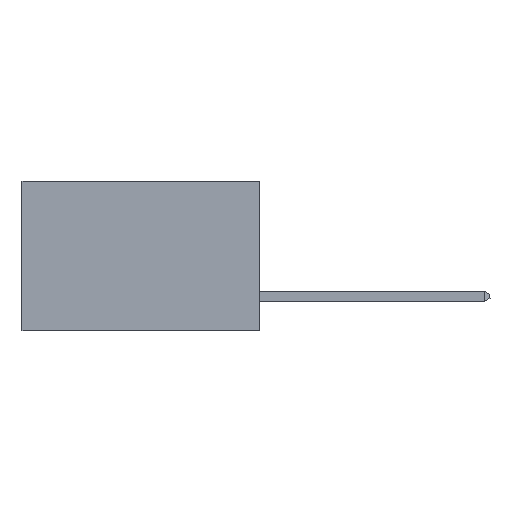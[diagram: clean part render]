
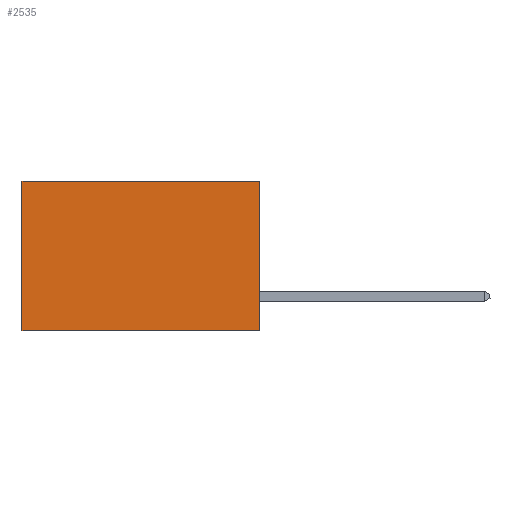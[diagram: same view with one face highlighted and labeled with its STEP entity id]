
A CAD part, left-side view. The second image highlights one B-rep face of the part: STEP entity #2535.
In plain terms, the highlighted planar face has unit normal (-1, 0, 0).
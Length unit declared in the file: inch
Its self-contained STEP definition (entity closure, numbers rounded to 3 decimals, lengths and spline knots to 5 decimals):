
#740 = VECTOR ( 'NONE', #2702, 39.37008 ) ;
#1398 = AXIS2_PLACEMENT_3D ( 'NONE', #10653, #1428, #5856 ) ;
#1407 = ORIENTED_EDGE ( 'NONE', *, *, #13389, .T. ) ;
#1428 = DIRECTION ( 'NONE',  ( 1., 0., 0. ) ) ;
#1784 = DIRECTION ( 'NONE',  ( 0., 1., 0. ) ) ;
#2108 = EDGE_CURVE ( 'NONE', #3399, #7770, #3367, .T. ) ;
#2535 = ADVANCED_FACE ( 'NONE', ( #5545 ), #6294, .F. ) ;
#2702 = DIRECTION ( 'NONE',  ( 0., 0., -1. ) ) ;
#2729 = VECTOR ( 'NONE', #1784, 39.37008 ) ;
#3332 = CARTESIAN_POINT ( 'NONE',  ( 0.277, 0.59, -0.37 ) ) ;
#3367 = LINE ( 'NONE', #5558, #4013 ) ;
#3399 = VERTEX_POINT ( 'NONE', #13139 ) ;
#3533 = DIRECTION ( 'NONE',  ( 0., 1., 0. ) ) ;
#3624 = LINE ( 'NONE', #6316, #740 ) ;
#4013 = VECTOR ( 'NONE', #3533, 39.37008 ) ;
#4144 = EDGE_CURVE ( 'NONE', #13652, #3399, #3624, .T. ) ;
#5545 = FACE_OUTER_BOUND ( 'NONE', #10223, .T. ) ;
#5558 = CARTESIAN_POINT ( 'NONE',  ( 0.277, 0., -0.37 ) ) ;
#5582 = LINE ( 'NONE', #12353, #2729 ) ;
#5856 = DIRECTION ( 'NONE',  ( 0., 0., -1. ) ) ;
#6294 = PLANE ( 'NONE',  #1398 ) ;
#6316 = CARTESIAN_POINT ( 'NONE',  ( 0.277, 0., -0.37 ) ) ;
#7189 = LINE ( 'NONE', #3332, #10255 ) ;
#7770 = VERTEX_POINT ( 'NONE', #10559 ) ;
#8631 = DIRECTION ( 'NONE',  ( 0., 0., -1. ) ) ;
#8984 = CARTESIAN_POINT ( 'NONE',  ( 0.277, 0., 0. ) ) ;
#10072 = CARTESIAN_POINT ( 'NONE',  ( 0.277, 0.59, 0. ) ) ;
#10223 = EDGE_LOOP ( 'NONE', ( #1407, #11291, #11586, #13709 ) ) ;
#10255 = VECTOR ( 'NONE', #8631, 39.37008 ) ;
#10559 = CARTESIAN_POINT ( 'NONE',  ( 0.277, 0.59, -0.37 ) ) ;
#10653 = CARTESIAN_POINT ( 'NONE',  ( 0.277, 0., -0.37 ) ) ;
#11188 = EDGE_CURVE ( 'NONE', #13652, #11852, #5582, .T. ) ;
#11291 = ORIENTED_EDGE ( 'NONE', *, *, #2108, .F. ) ;
#11586 = ORIENTED_EDGE ( 'NONE', *, *, #4144, .F. ) ;
#11852 = VERTEX_POINT ( 'NONE', #10072 ) ;
#12353 = CARTESIAN_POINT ( 'NONE',  ( 0.277, 0., 0. ) ) ;
#13139 = CARTESIAN_POINT ( 'NONE',  ( 0.277, 0., -0.37 ) ) ;
#13389 = EDGE_CURVE ( 'NONE', #11852, #7770, #7189, .T. ) ;
#13652 = VERTEX_POINT ( 'NONE', #8984 ) ;
#13709 = ORIENTED_EDGE ( 'NONE', *, *, #11188, .T. ) ;
